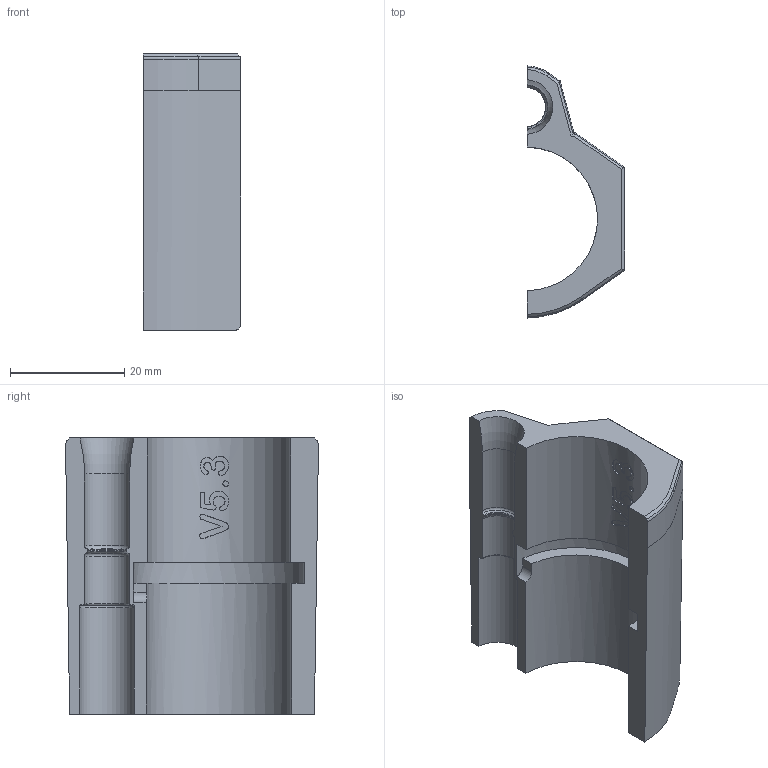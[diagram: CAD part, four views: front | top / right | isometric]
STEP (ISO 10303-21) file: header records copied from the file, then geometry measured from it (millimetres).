
FILE_DESCRIPTION (( 'STEP AP203' ), '1' );
FILE_NAME ('Orca Barrel Mount Left V5.3.STEP', '2023-01-20T23:41:59', ( '' ), ( '' ), 'SwSTEP 2.0', 'SolidWorks 2021', '' );
FILE_SCHEMA (( 'CONFIG_CONTROL_DESIGN' ));
Length unit declared in the file: inch
Products named in the file (1): Orca Barrel Mount Left V5.3
Bounding box: 17.09 x 44.11 x 48.34 mm (x, y, z)
Volume: 12348.3 mm3; surface area: 6780.2 mm2
Topology: 1 solids, 1 shells, 120 faces, 331 edges, 217 vertices
Faces by surface type: bspline 56, plane 26, cylinder 22, torus 11, cone 5
Entity records: 11454 total; most frequent: CARTESIAN_POINT 8879, ORIENTED_EDGE 662, EDGE_CURVE 331, DIRECTION 289, VERTEX_POINT 217, B_SPLINE_CURVE_WITH_KNOTS 200, EDGE_LOOP 124, ADVANCED_FACE 120
